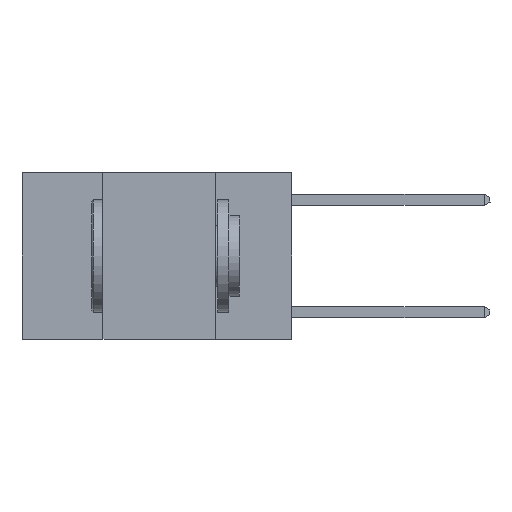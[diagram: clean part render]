
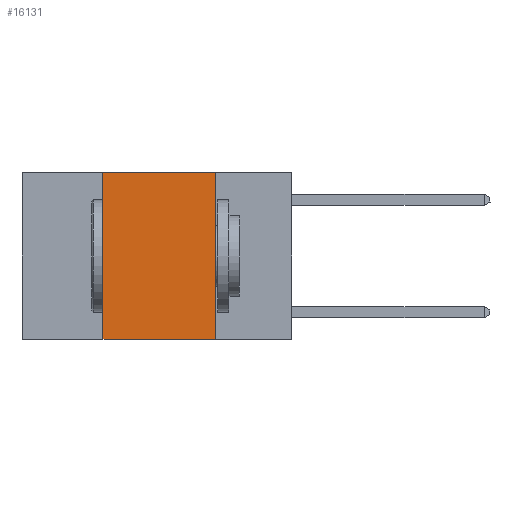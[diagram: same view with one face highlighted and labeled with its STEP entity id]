
A CAD part, left-side view. The second image highlights one B-rep face of the part: STEP entity #16131.
In plain terms, the highlighted planar face has unit normal (-1, 0, 0).
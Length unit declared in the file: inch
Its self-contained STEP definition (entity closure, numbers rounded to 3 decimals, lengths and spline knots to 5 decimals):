
#462 = PLANE ( 'NONE',  #14194 ) ;
#797 = CARTESIAN_POINT ( 'NONE',  ( 0., 0.6, 0. ) ) ;
#915 = DIRECTION ( 'NONE',  ( 0., -1., 0. ) ) ;
#1504 = CARTESIAN_POINT ( 'NONE',  ( 0., 0.17, 0. ) ) ;
#1629 = CARTESIAN_POINT ( 'NONE',  ( 0., 0.6, 0. ) ) ;
#2332 = ORIENTED_EDGE ( 'NONE', *, *, #6433, .F. ) ;
#2534 = VERTEX_POINT ( 'NONE', #17487 ) ;
#2571 = EDGE_CURVE ( 'NONE', #14253, #7483, #8114, .T. ) ;
#2876 = LINE ( 'NONE', #9833, #14067 ) ;
#4369 = EDGE_LOOP ( 'NONE', ( #15735, #12193, #2332, #16510 ) ) ;
#5510 = EDGE_CURVE ( 'NONE', #16734, #7483, #6806, .T. ) ;
#5787 = FACE_OUTER_BOUND ( 'NONE', #4369, .T. ) ;
#6433 = EDGE_CURVE ( 'NONE', #14253, #2534, #2876, .T. ) ;
#6806 = LINE ( 'NONE', #1504, #15786 ) ;
#7210 = DIRECTION ( 'NONE',  ( 1., 0., 0. ) ) ;
#7483 = VERTEX_POINT ( 'NONE', #16974 ) ;
#7536 = CARTESIAN_POINT ( 'NONE',  ( 0., 0.17, 0. ) ) ;
#8078 = DIRECTION ( 'NONE',  ( 0., 0., -1. ) ) ;
#8114 = LINE ( 'NONE', #9136, #12111 ) ;
#8283 = DIRECTION ( 'NONE',  ( 0., 0., 1. ) ) ;
#9136 = CARTESIAN_POINT ( 'NONE',  ( 0., 0.6, -0.37 ) ) ;
#9661 = VECTOR ( 'NONE', #11684, 39.37008 ) ;
#9833 = CARTESIAN_POINT ( 'NONE',  ( 0., 0.42, 0. ) ) ;
#10860 = CARTESIAN_POINT ( 'NONE',  ( 0., 0.42, -0.37 ) ) ;
#11684 = DIRECTION ( 'NONE',  ( 0., -1., 0. ) ) ;
#12111 = VECTOR ( 'NONE', #915, 39.37008 ) ;
#12193 = ORIENTED_EDGE ( 'NONE', *, *, #16792, .F. ) ;
#14067 = VECTOR ( 'NONE', #8283, 39.37008 ) ;
#14194 = AXIS2_PLACEMENT_3D ( 'NONE', #1629, #7210, #15405 ) ;
#14253 = VERTEX_POINT ( 'NONE', #10860 ) ;
#15405 = DIRECTION ( 'NONE',  ( 0., 0., -1. ) ) ;
#15651 = LINE ( 'NONE', #797, #9661 ) ;
#15735 = ORIENTED_EDGE ( 'NONE', *, *, #5510, .F. ) ;
#15786 = VECTOR ( 'NONE', #8078, 39.37008 ) ;
#16131 = ADVANCED_FACE ( 'NONE', ( #5787 ), #462, .F. ) ;
#16510 = ORIENTED_EDGE ( 'NONE', *, *, #2571, .T. ) ;
#16734 = VERTEX_POINT ( 'NONE', #7536 ) ;
#16792 = EDGE_CURVE ( 'NONE', #2534, #16734, #15651, .T. ) ;
#16974 = CARTESIAN_POINT ( 'NONE',  ( 0., 0.17, -0.37 ) ) ;
#17487 = CARTESIAN_POINT ( 'NONE',  ( 0., 0.42, 0. ) ) ;
